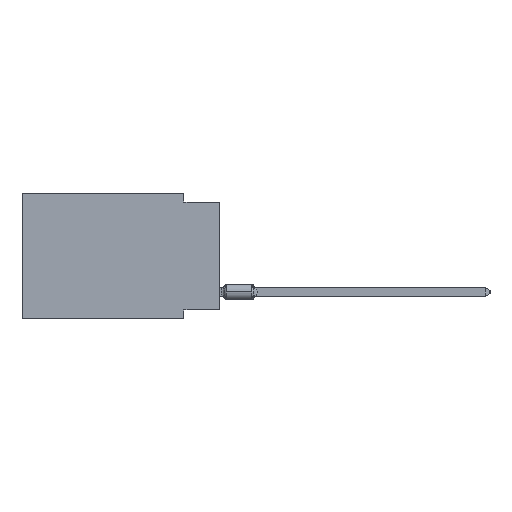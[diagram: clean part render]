
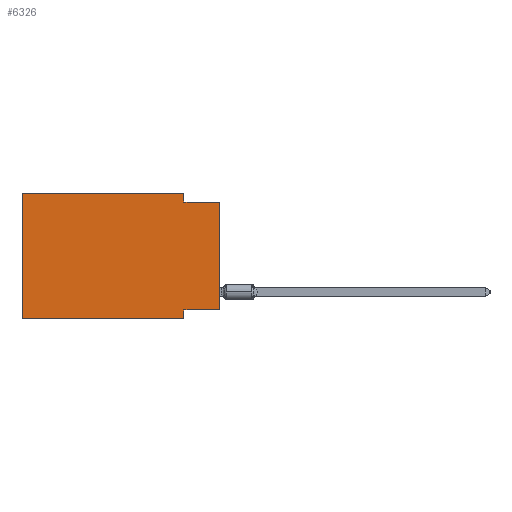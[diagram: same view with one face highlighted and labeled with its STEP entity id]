
A CAD part, left-side view. The second image highlights one B-rep face of the part: STEP entity #6326.
In plain terms, the highlighted planar face has unit normal (-1, 0, 0).
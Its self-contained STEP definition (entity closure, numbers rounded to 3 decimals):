
#472 = LINE ( 'NONE', #22445, #39992 ) ;
#1340 = CARTESIAN_POINT ( 'NONE',  ( 0., 2.54, 0. ) ) ;
#1632 = LINE ( 'NONE', #1340, #4793 ) ;
#2306 = DIRECTION ( 'NONE',  ( 0., -1., 0. ) ) ;
#2504 = VECTOR ( 'NONE', #44364, 1000. ) ;
#2701 = ORIENTED_EDGE ( 'NONE', *, *, #42352, .F. ) ;
#2799 = DIRECTION ( 'NONE',  ( 0., 1., 0. ) ) ;
#3081 = CARTESIAN_POINT ( 'NONE',  ( 0., 0., -8.255 ) ) ;
#4464 = LINE ( 'NONE', #43220, #2504 ) ;
#4704 = VERTEX_POINT ( 'NONE', #35597 ) ;
#4793 = VECTOR ( 'NONE', #19826, 1000. ) ;
#5721 = VERTEX_POINT ( 'NONE', #20383 ) ;
#6326 = ADVANCED_FACE ( 'NONE', ( #12506 ), #51550, .F. ) ;
#7230 = ORIENTED_EDGE ( 'NONE', *, *, #32704, .T. ) ;
#7595 = DIRECTION ( 'NONE',  ( 1., 0., 0. ) ) ;
#7848 = CARTESIAN_POINT ( 'NONE',  ( 0., 13.97, 0. ) ) ;
#8546 = ORIENTED_EDGE ( 'NONE', *, *, #54973, .F. ) ;
#9443 = DIRECTION ( 'NONE',  ( 0., 0., 1. ) ) ;
#10418 = VERTEX_POINT ( 'NONE', #11209 ) ;
#11209 = CARTESIAN_POINT ( 'NONE',  ( 0., 2.54, 0. ) ) ;
#11934 = CARTESIAN_POINT ( 'NONE',  ( 0., 13.97, 0. ) ) ;
#12506 = FACE_OUTER_BOUND ( 'NONE', #47154, .T. ) ;
#13801 = VECTOR ( 'NONE', #2306, 1000. ) ;
#13806 = EDGE_CURVE ( 'NONE', #10418, #30896, #1632, .T. ) ;
#14606 = CARTESIAN_POINT ( 'NONE',  ( 0., 13.97, 0. ) ) ;
#14648 = ORIENTED_EDGE ( 'NONE', *, *, #13806, .F. ) ;
#16963 = VECTOR ( 'NONE', #24707, 1000. ) ;
#17652 = EDGE_CURVE ( 'NONE', #24180, #27026, #24184, .T. ) ;
#19826 = DIRECTION ( 'NONE',  ( 0., 0., -1. ) ) ;
#20383 = CARTESIAN_POINT ( 'NONE',  ( 0., 13.97, -8.89 ) ) ;
#20890 = ORIENTED_EDGE ( 'NONE', *, *, #37721, .T. ) ;
#22445 = CARTESIAN_POINT ( 'NONE',  ( 0., 0., 0. ) ) ;
#24180 = VERTEX_POINT ( 'NONE', #3081 ) ;
#24184 = LINE ( 'NONE', #24472, #25300 ) ;
#24472 = CARTESIAN_POINT ( 'NONE',  ( 0., 0., -8.255 ) ) ;
#24707 = DIRECTION ( 'NONE',  ( 0., -1., 0. ) ) ;
#25109 = VERTEX_POINT ( 'NONE', #7848 ) ;
#25300 = VECTOR ( 'NONE', #2799, 1000. ) ;
#25540 = ORIENTED_EDGE ( 'NONE', *, *, #53191, .F. ) ;
#25801 = DIRECTION ( 'NONE',  ( 0., 0., -1. ) ) ;
#27026 = VERTEX_POINT ( 'NONE', #37095 ) ;
#27409 = CARTESIAN_POINT ( 'NONE',  ( 0., 13.97, -8.89 ) ) ;
#27911 = LINE ( 'NONE', #41777, #49429 ) ;
#28510 = CARTESIAN_POINT ( 'NONE',  ( 0., 2.54, -8.89 ) ) ;
#30896 = VERTEX_POINT ( 'NONE', #36850 ) ;
#32704 = EDGE_CURVE ( 'NONE', #5721, #55892, #49388, .T. ) ;
#35597 = CARTESIAN_POINT ( 'NONE',  ( 0., 0., -0.635 ) ) ;
#35778 = ORIENTED_EDGE ( 'NONE', *, *, #17652, .F. ) ;
#36583 = LINE ( 'NONE', #14606, #16963 ) ;
#36600 = DIRECTION ( 'NONE',  ( 0., 0., -1. ) ) ;
#36850 = CARTESIAN_POINT ( 'NONE',  ( 0., 2.54, -0.635 ) ) ;
#37095 = CARTESIAN_POINT ( 'NONE',  ( 0., 2.54, -8.255 ) ) ;
#37294 = CARTESIAN_POINT ( 'NONE',  ( 0., 0., -0.635 ) ) ;
#37721 = EDGE_CURVE ( 'NONE', #24180, #4704, #472, .T. ) ;
#38118 = EDGE_CURVE ( 'NONE', #25109, #10418, #36583, .T. ) ;
#38389 = AXIS2_PLACEMENT_3D ( 'NONE', #11934, #7595, #25801 ) ;
#39059 = ORIENTED_EDGE ( 'NONE', *, *, #38118, .F. ) ;
#39992 = VECTOR ( 'NONE', #9443, 1000. ) ;
#41777 = CARTESIAN_POINT ( 'NONE',  ( 0., 2.54, -8.89 ) ) ;
#42352 = EDGE_CURVE ( 'NONE', #27026, #55892, #27911, .T. ) ;
#43220 = CARTESIAN_POINT ( 'NONE',  ( 0., 13.97, 0. ) ) ;
#44341 = VECTOR ( 'NONE', #45045, 1000. ) ;
#44364 = DIRECTION ( 'NONE',  ( 0., 0., 1. ) ) ;
#45045 = DIRECTION ( 'NONE',  ( 0., -1., 0. ) ) ;
#47154 = EDGE_LOOP ( 'NONE', ( #20890, #25540, #14648, #39059, #8546, #7230, #2701, #35778 ) ) ;
#49388 = LINE ( 'NONE', #27409, #44341 ) ;
#49429 = VECTOR ( 'NONE', #36600, 1000. ) ;
#50312 = LINE ( 'NONE', #37294, #13801 ) ;
#51550 = PLANE ( 'NONE',  #38389 ) ;
#53191 = EDGE_CURVE ( 'NONE', #30896, #4704, #50312, .T. ) ;
#54973 = EDGE_CURVE ( 'NONE', #5721, #25109, #4464, .T. ) ;
#55892 = VERTEX_POINT ( 'NONE', #28510 ) ;
